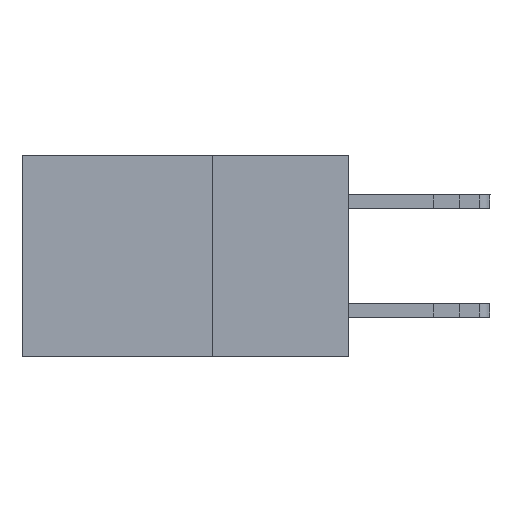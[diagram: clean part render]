
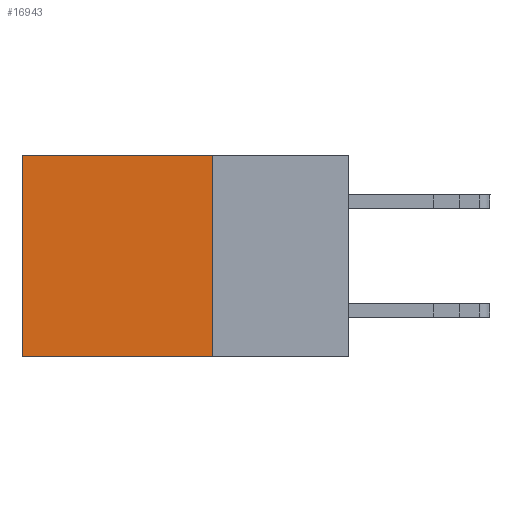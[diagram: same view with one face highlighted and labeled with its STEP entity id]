
A CAD part, left-side view. The second image highlights one B-rep face of the part: STEP entity #16943.
In plain terms, the highlighted planar face has unit normal (-1, 0, 0).
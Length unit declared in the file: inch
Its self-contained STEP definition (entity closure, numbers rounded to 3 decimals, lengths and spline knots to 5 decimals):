
#565 = FACE_OUTER_BOUND ( 'NONE', #16478, .T. ) ;
#695 = VECTOR ( 'NONE', #9952, 39.37008 ) ;
#2767 = AXIS2_PLACEMENT_3D ( 'NONE', #8641, #3725, #14824 ) ;
#3381 = VECTOR ( 'NONE', #14201, 39.37008 ) ;
#3693 = CARTESIAN_POINT ( 'NONE',  ( 0.298, 0.25, -0.37 ) ) ;
#3725 = DIRECTION ( 'NONE',  ( 1., 0., 0. ) ) ;
#5016 = VERTEX_POINT ( 'NONE', #19176 ) ;
#5331 = LINE ( 'NONE', #3693, #695 ) ;
#5375 = ORIENTED_EDGE ( 'NONE', *, *, #11914, .T. ) ;
#6326 = LINE ( 'NONE', #11059, #16804 ) ;
#7041 = CARTESIAN_POINT ( 'NONE',  ( 0.298, 0.6, 0. ) ) ;
#7161 = VERTEX_POINT ( 'NONE', #9253 ) ;
#8338 = PLANE ( 'NONE',  #2767 ) ;
#8641 = CARTESIAN_POINT ( 'NONE',  ( 0.298, 0.25, 0. ) ) ;
#9061 = VERTEX_POINT ( 'NONE', #10255 ) ;
#9253 = CARTESIAN_POINT ( 'NONE',  ( 0.298, 0.25, -0.37 ) ) ;
#9952 = DIRECTION ( 'NONE',  ( 0., 1., 0. ) ) ;
#10255 = CARTESIAN_POINT ( 'NONE',  ( 0.298, 0.25, 0. ) ) ;
#10405 = EDGE_CURVE ( 'NONE', #7161, #5016, #5331, .T. ) ;
#11025 = CARTESIAN_POINT ( 'NONE',  ( 0.298, 0.25, 0. ) ) ;
#11059 = CARTESIAN_POINT ( 'NONE',  ( 0.298, 0.25, 0. ) ) ;
#11914 = EDGE_CURVE ( 'NONE', #11956, #5016, #19448, .T. ) ;
#11956 = VERTEX_POINT ( 'NONE', #7041 ) ;
#12995 = ORIENTED_EDGE ( 'NONE', *, *, #10405, .F. ) ;
#13171 = EDGE_CURVE ( 'NONE', #9061, #7161, #6326, .T. ) ;
#13193 = CARTESIAN_POINT ( 'NONE',  ( 0.298, 0.6, 0. ) ) ;
#13682 = DIRECTION ( 'NONE',  ( 0., 0., -1. ) ) ;
#13833 = VECTOR ( 'NONE', #13682, 39.37008 ) ;
#14132 = ORIENTED_EDGE ( 'NONE', *, *, #13171, .F. ) ;
#14201 = DIRECTION ( 'NONE',  ( 0., 1., 0. ) ) ;
#14824 = DIRECTION ( 'NONE',  ( 0., 0., -1. ) ) ;
#15610 = EDGE_CURVE ( 'NONE', #9061, #11956, #15839, .T. ) ;
#15839 = LINE ( 'NONE', #11025, #3381 ) ;
#16478 = EDGE_LOOP ( 'NONE', ( #5375, #12995, #14132, #18455 ) ) ;
#16804 = VECTOR ( 'NONE', #17315, 39.37008 ) ;
#16943 = ADVANCED_FACE ( 'NONE', ( #565 ), #8338, .F. ) ;
#17315 = DIRECTION ( 'NONE',  ( 0., 0., -1. ) ) ;
#18455 = ORIENTED_EDGE ( 'NONE', *, *, #15610, .T. ) ;
#19176 = CARTESIAN_POINT ( 'NONE',  ( 0.298, 0.6, -0.37 ) ) ;
#19448 = LINE ( 'NONE', #13193, #13833 ) ;
